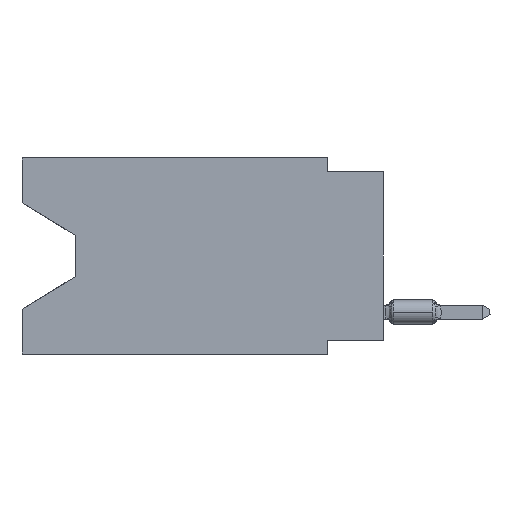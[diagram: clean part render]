
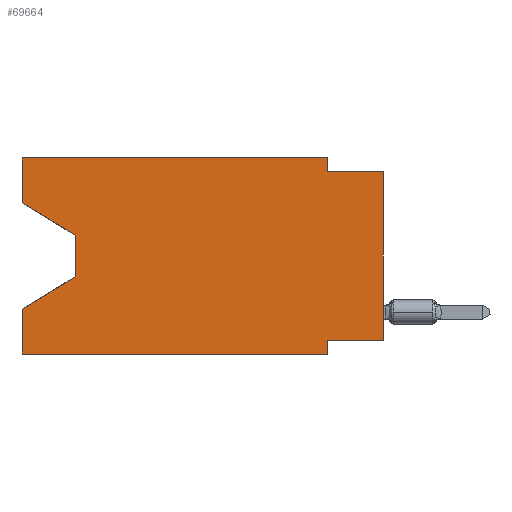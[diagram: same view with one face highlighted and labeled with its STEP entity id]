
A CAD part, left-side view. The second image highlights one B-rep face of the part: STEP entity #69664.
In plain terms, the highlighted planar face has unit normal (-1, 0, 0).
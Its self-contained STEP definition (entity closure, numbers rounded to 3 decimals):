
#3400 = EDGE_CURVE ( 'NONE', #33081, #26256, #50909, .T. ) ;
#3675 = DIRECTION ( 'NONE',  ( 0., 0., -1. ) ) ;
#4165 = ORIENTED_EDGE ( 'NONE', *, *, #54935, .T. ) ;
#4212 = LINE ( 'NONE', #5002, #12948 ) ;
#5002 = CARTESIAN_POINT ( 'NONE',  ( 0., 16.383, 0. ) ) ;
#8217 = LINE ( 'NONE', #32432, #64182 ) ;
#10421 = LINE ( 'NONE', #64791, #15382 ) ;
#11795 = EDGE_CURVE ( 'NONE', #65769, #25040, #10421, .T. ) ;
#12458 = CARTESIAN_POINT ( 'NONE',  ( 0., 16.383, 0. ) ) ;
#12948 = VECTOR ( 'NONE', #71258, 1000. ) ;
#13919 = VERTEX_POINT ( 'NONE', #20986 ) ;
#14299 = EDGE_CURVE ( 'NONE', #51442, #25040, #4212, .T. ) ;
#14795 = DIRECTION ( 'NONE',  ( 0., -1., 0. ) ) ;
#15382 = VECTOR ( 'NONE', #69566, 1000. ) ;
#15645 = CARTESIAN_POINT ( 'NONE',  ( 0., 2.54, -8.255 ) ) ;
#16178 = VECTOR ( 'NONE', #3675, 1000. ) ;
#16609 = VERTEX_POINT ( 'NONE', #32263 ) ;
#17000 = EDGE_LOOP ( 'NONE', ( #4165, #31051, #18120, #69010, #47268, #36223, #37291, #39647, #69888, #60404, #21878, #41008 ) ) ;
#18120 = ORIENTED_EDGE ( 'NONE', *, *, #11795, .T. ) ;
#20423 = CARTESIAN_POINT ( 'NONE',  ( 0., 0., 0. ) ) ;
#20986 = CARTESIAN_POINT ( 'NONE',  ( 0., 16.383, -2.038 ) ) ;
#21150 = LINE ( 'NONE', #40187, #25133 ) ;
#21878 = ORIENTED_EDGE ( 'NONE', *, *, #3400, .F. ) ;
#22405 = DIRECTION ( 'NONE',  ( 0., -0.855, -0.519 ) ) ;
#24234 = PLANE ( 'NONE',  #28506 ) ;
#24614 = CARTESIAN_POINT ( 'NONE',  ( 0., 16.383, 0. ) ) ;
#25040 = VERTEX_POINT ( 'NONE', #75095 ) ;
#25133 = VECTOR ( 'NONE', #64372, 1000. ) ;
#25940 = CARTESIAN_POINT ( 'NONE',  ( 0., 2.54, -0.635 ) ) ;
#26256 = VERTEX_POINT ( 'NONE', #30344 ) ;
#27705 = EDGE_CURVE ( 'NONE', #51442, #33030, #8217, .T. ) ;
#28506 = AXIS2_PLACEMENT_3D ( 'NONE', #24614, #29780, #35735 ) ;
#29017 = CARTESIAN_POINT ( 'NONE',  ( 0., 13.97, -3.505 ) ) ;
#29780 = DIRECTION ( 'NONE',  ( 1., 0., 0. ) ) ;
#29862 = EDGE_CURVE ( 'NONE', #16609, #39741, #21150, .T. ) ;
#29936 = VECTOR ( 'NONE', #60815, 1000. ) ;
#30344 = CARTESIAN_POINT ( 'NONE',  ( 0., 2.54, 0. ) ) ;
#30565 = FACE_OUTER_BOUND ( 'NONE', #17000, .T. ) ;
#31051 = ORIENTED_EDGE ( 'NONE', *, *, #51919, .T. ) ;
#32263 = CARTESIAN_POINT ( 'NONE',  ( 0., 0., -8.255 ) ) ;
#32398 = VECTOR ( 'NONE', #43871, 1000. ) ;
#32432 = CARTESIAN_POINT ( 'NONE',  ( 0., 16.383, -8.89 ) ) ;
#33030 = VERTEX_POINT ( 'NONE', #35497 ) ;
#33081 = VERTEX_POINT ( 'NONE', #12458 ) ;
#33896 = CARTESIAN_POINT ( 'NONE',  ( 0., 16.383, -2.038 ) ) ;
#35091 = LINE ( 'NONE', #33896, #66769 ) ;
#35497 = CARTESIAN_POINT ( 'NONE',  ( 0., 2.54, -8.89 ) ) ;
#35735 = DIRECTION ( 'NONE',  ( 0., 0., -1. ) ) ;
#36223 = ORIENTED_EDGE ( 'NONE', *, *, #72331, .F. ) ;
#37291 = ORIENTED_EDGE ( 'NONE', *, *, #29862, .F. ) ;
#39647 = ORIENTED_EDGE ( 'NONE', *, *, #59947, .T. ) ;
#39741 = VERTEX_POINT ( 'NONE', #15645 ) ;
#40187 = CARTESIAN_POINT ( 'NONE',  ( 0., 0., -8.255 ) ) ;
#40739 = CARTESIAN_POINT ( 'NONE',  ( 0., 16.383, -8.89 ) ) ;
#41008 = ORIENTED_EDGE ( 'NONE', *, *, #54845, .F. ) ;
#42506 = CARTESIAN_POINT ( 'NONE',  ( 0., 13.97, -3.505 ) ) ;
#43755 = CARTESIAN_POINT ( 'NONE',  ( 0., 0., -0.635 ) ) ;
#43871 = DIRECTION ( 'NONE',  ( 0., 0., 1. ) ) ;
#44966 = CARTESIAN_POINT ( 'NONE',  ( 0., 16.383, 0. ) ) ;
#45945 = VERTEX_POINT ( 'NONE', #25940 ) ;
#47200 = CARTESIAN_POINT ( 'NONE',  ( 0., 2.54, -8.89 ) ) ;
#47268 = ORIENTED_EDGE ( 'NONE', *, *, #27705, .T. ) ;
#47295 = LINE ( 'NONE', #42506, #61333 ) ;
#47353 = VECTOR ( 'NONE', #71383, 1000. ) ;
#47463 = VERTEX_POINT ( 'NONE', #63894 ) ;
#50588 = LINE ( 'NONE', #75953, #64204 ) ;
#50909 = LINE ( 'NONE', #44966, #51356 ) ;
#51356 = VECTOR ( 'NONE', #14795, 1000. ) ;
#51442 = VERTEX_POINT ( 'NONE', #40739 ) ;
#51919 = EDGE_CURVE ( 'NONE', #59421, #65769, #47295, .T. ) ;
#53939 = LINE ( 'NONE', #47200, #47353 ) ;
#54845 = EDGE_CURVE ( 'NONE', #13919, #33081, #50588, .T. ) ;
#54935 = EDGE_CURVE ( 'NONE', #13919, #59421, #35091, .T. ) ;
#56600 = EDGE_CURVE ( 'NONE', #26256, #45945, #76649, .T. ) ;
#56636 = DIRECTION ( 'NONE',  ( 0., -1., 0. ) ) ;
#58033 = CARTESIAN_POINT ( 'NONE',  ( 0., 2.54, 0. ) ) ;
#59421 = VERTEX_POINT ( 'NONE', #29017 ) ;
#59947 = EDGE_CURVE ( 'NONE', #16609, #47463, #62092, .T. ) ;
#60404 = ORIENTED_EDGE ( 'NONE', *, *, #56600, .F. ) ;
#60815 = DIRECTION ( 'NONE',  ( 0., -1., 0. ) ) ;
#61333 = VECTOR ( 'NONE', #66698, 1000. ) ;
#61729 = EDGE_CURVE ( 'NONE', #45945, #47463, #73505, .T. ) ;
#62092 = LINE ( 'NONE', #20423, #32398 ) ;
#62866 = DIRECTION ( 'NONE',  ( 0., 0., 1. ) ) ;
#63894 = CARTESIAN_POINT ( 'NONE',  ( 0., 0., -0.635 ) ) ;
#64182 = VECTOR ( 'NONE', #56636, 1000. ) ;
#64204 = VECTOR ( 'NONE', #62866, 1000. ) ;
#64372 = DIRECTION ( 'NONE',  ( 0., 1., 0. ) ) ;
#64791 = CARTESIAN_POINT ( 'NONE',  ( 0., 13.97, -5.385 ) ) ;
#65769 = VERTEX_POINT ( 'NONE', #77495 ) ;
#66698 = DIRECTION ( 'NONE',  ( 0., 0., -1. ) ) ;
#66769 = VECTOR ( 'NONE', #22405, 1000. ) ;
#69010 = ORIENTED_EDGE ( 'NONE', *, *, #14299, .F. ) ;
#69566 = DIRECTION ( 'NONE',  ( 0., 0.855, -0.519 ) ) ;
#69664 = ADVANCED_FACE ( 'NONE', ( #30565 ), #24234, .F. ) ;
#69888 = ORIENTED_EDGE ( 'NONE', *, *, #61729, .F. ) ;
#71258 = DIRECTION ( 'NONE',  ( 0., 0., 1. ) ) ;
#71383 = DIRECTION ( 'NONE',  ( 0., 0., -1. ) ) ;
#72331 = EDGE_CURVE ( 'NONE', #39741, #33030, #53939, .T. ) ;
#73505 = LINE ( 'NONE', #43755, #29936 ) ;
#75095 = CARTESIAN_POINT ( 'NONE',  ( 0., 16.383, -6.852 ) ) ;
#75953 = CARTESIAN_POINT ( 'NONE',  ( 0., 16.383, 0. ) ) ;
#76649 = LINE ( 'NONE', #58033, #16178 ) ;
#77495 = CARTESIAN_POINT ( 'NONE',  ( 0., 13.97, -5.385 ) ) ;
